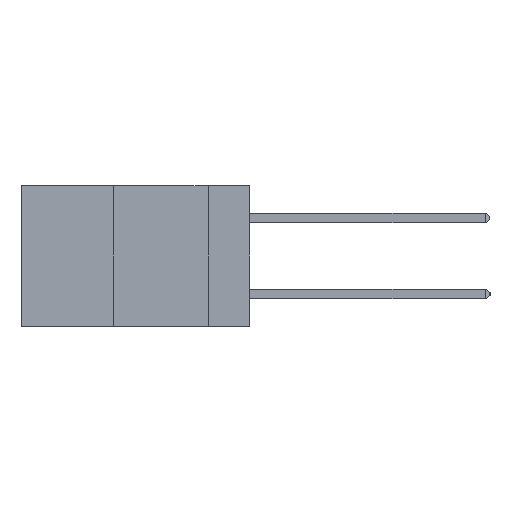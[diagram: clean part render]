
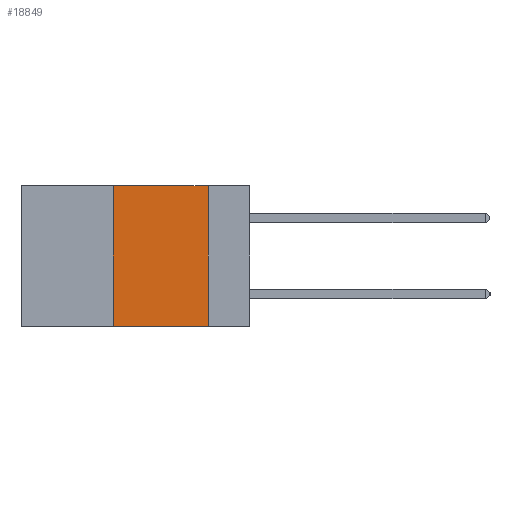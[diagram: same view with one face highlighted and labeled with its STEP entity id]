
A CAD part, left-side view. The second image highlights one B-rep face of the part: STEP entity #18849.
In plain terms, the highlighted planar face has unit normal (-1, 0, 0).
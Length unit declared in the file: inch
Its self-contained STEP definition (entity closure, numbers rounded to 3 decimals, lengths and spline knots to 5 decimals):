
#573 = VERTEX_POINT ( 'NONE', #1529 ) ;
#584 = LINE ( 'NONE', #9039, #9775 ) ;
#1104 = VECTOR ( 'NONE', #2514, 39.37008 ) ;
#1384 = ORIENTED_EDGE ( 'NONE', *, *, #8393, .F. ) ;
#1529 = CARTESIAN_POINT ( 'NONE',  ( 0., 0.36, -0.37 ) ) ;
#1868 = ORIENTED_EDGE ( 'NONE', *, *, #17280, .F. ) ;
#2262 = DIRECTION ( 'NONE',  ( 1., 0., 0. ) ) ;
#2378 = DIRECTION ( 'NONE',  ( 0., 0., -1. ) ) ;
#2514 = DIRECTION ( 'NONE',  ( 0., -1., 0. ) ) ;
#3298 = ORIENTED_EDGE ( 'NONE', *, *, #4295, .F. ) ;
#4295 = EDGE_CURVE ( 'NONE', #5872, #20706, #584, .T. ) ;
#5744 = ORIENTED_EDGE ( 'NONE', *, *, #15039, .T. ) ;
#5872 = VERTEX_POINT ( 'NONE', #15155 ) ;
#6669 = CARTESIAN_POINT ( 'NONE',  ( 0., 0.36, 0. ) ) ;
#6964 = CARTESIAN_POINT ( 'NONE',  ( 0., 0.36, 0. ) ) ;
#7351 = PLANE ( 'NONE',  #20914 ) ;
#7960 = VERTEX_POINT ( 'NONE', #6964 ) ;
#8059 = VECTOR ( 'NONE', #9920, 39.37008 ) ;
#8393 = EDGE_CURVE ( 'NONE', #7960, #5872, #17042, .T. ) ;
#8845 = CARTESIAN_POINT ( 'NONE',  ( 0., 0.11, -0.37 ) ) ;
#9039 = CARTESIAN_POINT ( 'NONE',  ( 0., 0.11, 0. ) ) ;
#9729 = LINE ( 'NONE', #12725, #1104 ) ;
#9775 = VECTOR ( 'NONE', #2378, 39.37008 ) ;
#9920 = DIRECTION ( 'NONE',  ( 0., -1., 0. ) ) ;
#10123 = LINE ( 'NONE', #6669, #18529 ) ;
#12471 = CARTESIAN_POINT ( 'NONE',  ( 0., 0.6, 0. ) ) ;
#12725 = CARTESIAN_POINT ( 'NONE',  ( 0., 0.6, -0.37 ) ) ;
#14207 = DIRECTION ( 'NONE',  ( 0., 0., -1. ) ) ;
#15039 = EDGE_CURVE ( 'NONE', #573, #20706, #9729, .T. ) ;
#15155 = CARTESIAN_POINT ( 'NONE',  ( 0., 0.11, 0. ) ) ;
#17042 = LINE ( 'NONE', #19866, #8059 ) ;
#17057 = EDGE_LOOP ( 'NONE', ( #3298, #1384, #1868, #5744 ) ) ;
#17280 = EDGE_CURVE ( 'NONE', #573, #7960, #10123, .T. ) ;
#18529 = VECTOR ( 'NONE', #20099, 39.37008 ) ;
#18849 = ADVANCED_FACE ( 'NONE', ( #20487 ), #7351, .F. ) ;
#19866 = CARTESIAN_POINT ( 'NONE',  ( 0., 0.6, 0. ) ) ;
#20099 = DIRECTION ( 'NONE',  ( 0., 0., 1. ) ) ;
#20487 = FACE_OUTER_BOUND ( 'NONE', #17057, .T. ) ;
#20706 = VERTEX_POINT ( 'NONE', #8845 ) ;
#20914 = AXIS2_PLACEMENT_3D ( 'NONE', #12471, #2262, #14207 ) ;
